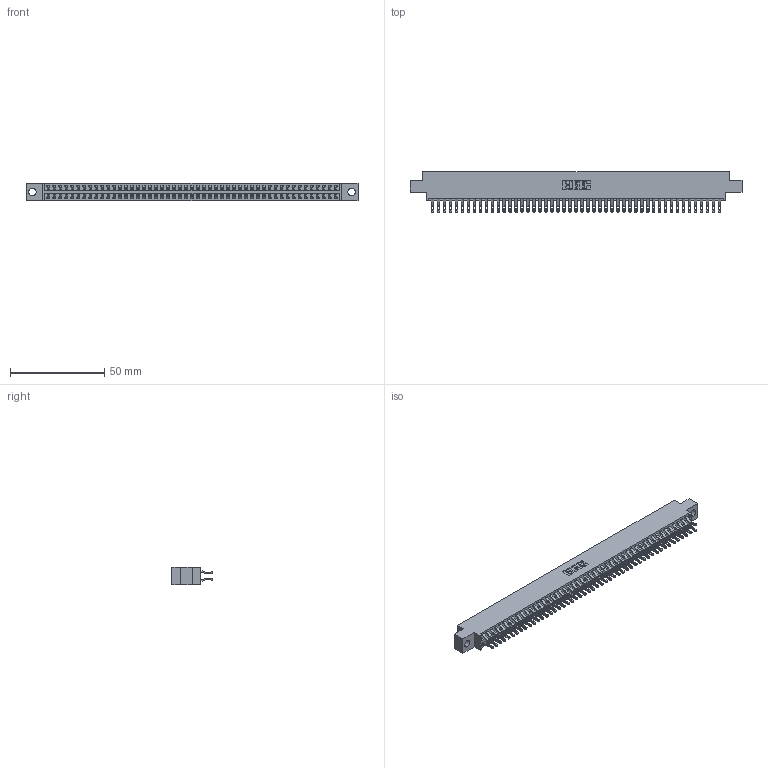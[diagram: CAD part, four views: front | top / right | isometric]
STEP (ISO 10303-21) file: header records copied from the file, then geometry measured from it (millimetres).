
FILE_DESCRIPTION (( 'STEP AP203' ), '1' );
FILE_NAME ('396-098-555-804.STEP', '2018-09-14T05:30:01', ( '' ), ( '' ), 'SwSTEP 2.0', 'SolidWorks 2016', '' );
FILE_SCHEMA (( 'CONFIG_CONTROL_DESIGN' ));
Length unit declared in the file: inch
Products named in the file (3): 346 Part_0.170 Offset - 0.156 Dia-TH; 345-292-001_555 Tail; 396-098-555-804
Assembly tree (99 placements, depth 2):
  396-098-555-804
    346 Part_0.170 Offset - 0.156 Dia-TH
    345-292-001_555 Tail  x98
Bounding box: 176.15 x 21.46 x 9.4 mm (x, y, z)
Volume: 17272.9 mm3; surface area: 24859 mm2
Topology: 99 solids, 99 shells, 5810 faces, 18275 edges, 12182 vertices
Faces by surface type: plane 3314, cylinder 2496
Entity records: 31497 total; most frequent: CARTESIAN_POINT 5218, ORIENTED_EDGE 5122, DIRECTION 4617, EDGE_CURVE 2561, LINE 2213, VECTOR 2213, VERTEX_POINT 1706, AXIS2_PLACEMENT_3D 1202
